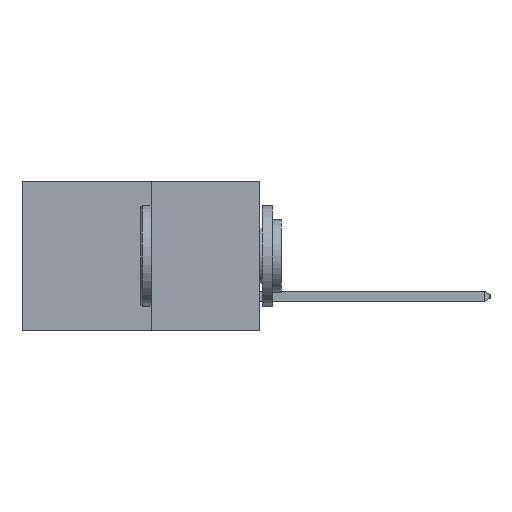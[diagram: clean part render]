
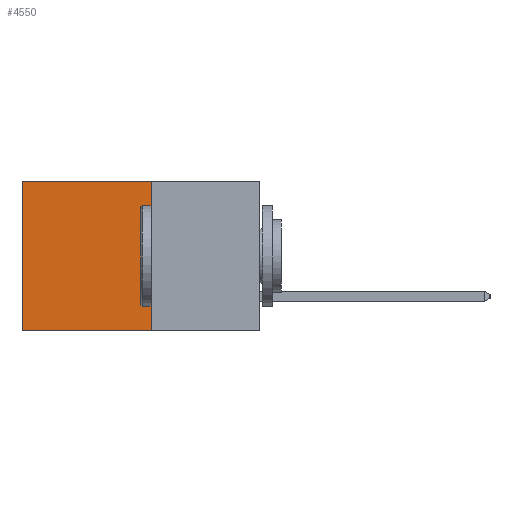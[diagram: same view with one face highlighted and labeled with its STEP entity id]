
A CAD part, left-side view. The second image highlights one B-rep face of the part: STEP entity #4550.
In plain terms, the highlighted planar face has unit normal (-1, 0, 0).
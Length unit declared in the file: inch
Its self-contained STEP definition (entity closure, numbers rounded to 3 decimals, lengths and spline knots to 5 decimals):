
#26 = VERTEX_POINT ( 'NONE', #12429 ) ;
#29 = EDGE_LOOP ( 'NONE', ( #749, #10318, #11709, #9339 ) ) ;
#161 = VECTOR ( 'NONE', #3159, 39.37008 ) ;
#556 = VERTEX_POINT ( 'NONE', #3266 ) ;
#749 = ORIENTED_EDGE ( 'NONE', *, *, #6924, .T. ) ;
#1486 = VECTOR ( 'NONE', #8305, 39.37008 ) ;
#2315 = VERTEX_POINT ( 'NONE', #9965 ) ;
#2948 = LINE ( 'NONE', #7278, #161 ) ;
#3124 = CARTESIAN_POINT ( 'NONE',  ( 0.277, 0.59, 0. ) ) ;
#3159 = DIRECTION ( 'NONE',  ( 0., 0., -1. ) ) ;
#3187 = VECTOR ( 'NONE', #10433, 39.37008 ) ;
#3266 = CARTESIAN_POINT ( 'NONE',  ( 0.277, 0.27, -0.37 ) ) ;
#4286 = LINE ( 'NONE', #5227, #1486 ) ;
#4363 = CARTESIAN_POINT ( 'NONE',  ( 0.277, 0.27, 0. ) ) ;
#4431 = DIRECTION ( 'NONE',  ( 0., 1., 0. ) ) ;
#4550 = ADVANCED_FACE ( 'NONE', ( #10243 ), #10084, .F. ) ;
#4999 = VECTOR ( 'NONE', #4431, 39.37008 ) ;
#5203 = EDGE_CURVE ( 'NONE', #2315, #6907, #8658, .T. ) ;
#5227 = CARTESIAN_POINT ( 'NONE',  ( 0.277, 0.59, -0.37 ) ) ;
#6483 = CARTESIAN_POINT ( 'NONE',  ( 0.277, 0.27, -0.37 ) ) ;
#6585 = AXIS2_PLACEMENT_3D ( 'NONE', #10100, #10755, #12840 ) ;
#6907 = VERTEX_POINT ( 'NONE', #3124 ) ;
#6924 = EDGE_CURVE ( 'NONE', #6907, #26, #4286, .T. ) ;
#7278 = CARTESIAN_POINT ( 'NONE',  ( 0.277, 0.27, -0.37 ) ) ;
#7716 = LINE ( 'NONE', #6483, #4999 ) ;
#8305 = DIRECTION ( 'NONE',  ( 0., 0., -1. ) ) ;
#8598 = EDGE_CURVE ( 'NONE', #2315, #556, #2948, .T. ) ;
#8658 = LINE ( 'NONE', #4363, #3187 ) ;
#9339 = ORIENTED_EDGE ( 'NONE', *, *, #5203, .T. ) ;
#9965 = CARTESIAN_POINT ( 'NONE',  ( 0.277, 0.27, 0. ) ) ;
#10084 = PLANE ( 'NONE',  #6585 ) ;
#10100 = CARTESIAN_POINT ( 'NONE',  ( 0.277, 0.27, -0.37 ) ) ;
#10243 = FACE_OUTER_BOUND ( 'NONE', #29, .T. ) ;
#10318 = ORIENTED_EDGE ( 'NONE', *, *, #11987, .F. ) ;
#10433 = DIRECTION ( 'NONE',  ( 0., 1., 0. ) ) ;
#10755 = DIRECTION ( 'NONE',  ( 1., 0., 0. ) ) ;
#11709 = ORIENTED_EDGE ( 'NONE', *, *, #8598, .F. ) ;
#11987 = EDGE_CURVE ( 'NONE', #556, #26, #7716, .T. ) ;
#12429 = CARTESIAN_POINT ( 'NONE',  ( 0.277, 0.59, -0.37 ) ) ;
#12840 = DIRECTION ( 'NONE',  ( 0., 0., -1. ) ) ;
